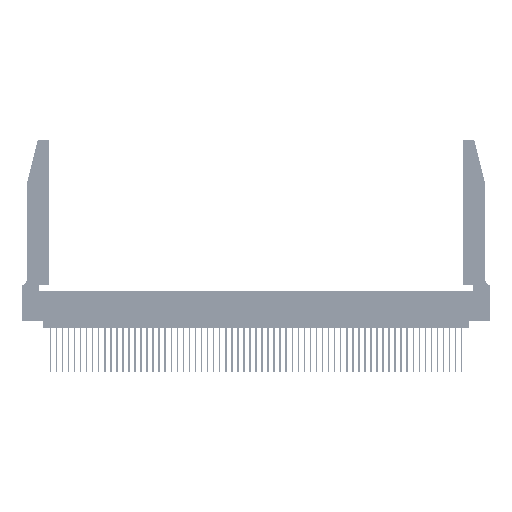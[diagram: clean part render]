
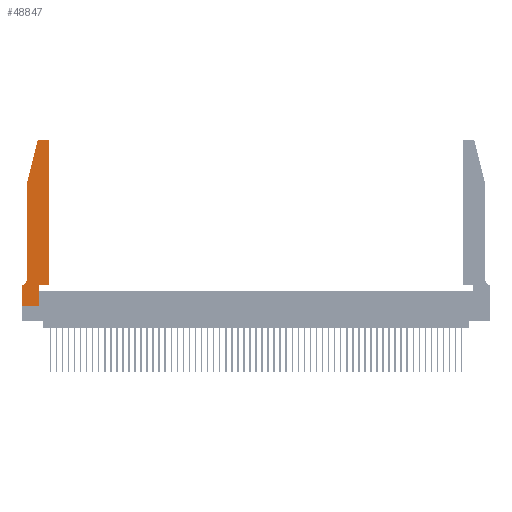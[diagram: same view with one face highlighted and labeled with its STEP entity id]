
A CAD part, top view. The second image highlights one B-rep face of the part: STEP entity #48847.
In plain terms, the highlighted planar face has unit normal (0, 0, 1).
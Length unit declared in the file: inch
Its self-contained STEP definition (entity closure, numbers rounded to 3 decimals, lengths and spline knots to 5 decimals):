
#72 = DIRECTION ( 'NONE',  ( 0., 0., 1. ) ) ;
#835 = CARTESIAN_POINT ( 'NONE',  ( 0.0755, 2., 0.37 ) ) ;
#942 = ORIENTED_EDGE ( 'NONE', *, *, #16438, .T. ) ;
#1132 = ORIENTED_EDGE ( 'NONE', *, *, #42555, .T. ) ;
#1268 = CIRCLE ( 'NONE', #54302, 0.03 ) ;
#1306 = DIRECTION ( 'NONE',  ( -1., 0., 0. ) ) ;
#1965 = CARTESIAN_POINT ( 'NONE',  ( 0.0755, 2., 0.37 ) ) ;
#4130 = ORIENTED_EDGE ( 'NONE', *, *, #50214, .T. ) ;
#4265 = CARTESIAN_POINT ( 'NONE',  ( 0.0055, 0.35, 0.37 ) ) ;
#4312 = VECTOR ( 'NONE', #8279, 39.37008 ) ;
#4739 = DIRECTION ( 'NONE',  ( 1., 0., 0. ) ) ;
#5356 = CARTESIAN_POINT ( 'NONE',  ( 0.4505, 0.35, 0.37 ) ) ;
#5868 = CARTESIAN_POINT ( 'NONE',  ( 0.2605, 2.75, 0.37 ) ) ;
#6295 = DIRECTION ( 'NONE',  ( 1., 0., 0. ) ) ;
#6496 = EDGE_CURVE ( 'NONE', #35958, #31170, #50195, .T. ) ;
#7111 = DIRECTION ( 'NONE',  ( 0., 1., 0. ) ) ;
#7503 = VECTOR ( 'NONE', #12842, 39.37008 ) ;
#8279 = DIRECTION ( 'NONE',  ( 0., -1., 0. ) ) ;
#8580 = DIRECTION ( 'NONE',  ( 1., 0., 0. ) ) ;
#9675 = EDGE_CURVE ( 'NONE', #44584, #35958, #25806, .T. ) ;
#10403 = ORIENTED_EDGE ( 'NONE', *, *, #6496, .T. ) ;
#10799 = VERTEX_POINT ( 'NONE', #4265 ) ;
#10897 = VERTEX_POINT ( 'NONE', #51812 ) ;
#11617 = VERTEX_POINT ( 'NONE', #24992 ) ;
#12486 = CARTESIAN_POINT ( 'NONE',  ( 0.4505, 0.35, 0.37 ) ) ;
#12708 = CARTESIAN_POINT ( 'NONE',  ( 0.4205, 2.72, 0.37 ) ) ;
#12842 = DIRECTION ( 'NONE',  ( 1., 0., 0. ) ) ;
#13895 = VERTEX_POINT ( 'NONE', #17860 ) ;
#15445 = DIRECTION ( 'NONE',  ( 0., 0., 1. ) ) ;
#15878 = DIRECTION ( 'NONE',  ( -1., 0., 0. ) ) ;
#16294 = ORIENTED_EDGE ( 'NONE', *, *, #53197, .T. ) ;
#16438 = EDGE_CURVE ( 'NONE', #42664, #13895, #1268, .T. ) ;
#17844 = VERTEX_POINT ( 'NONE', #43157 ) ;
#17860 = CARTESIAN_POINT ( 'NONE',  ( 0.4205, 2.75, 0.37 ) ) ;
#18050 = VECTOR ( 'NONE', #21969, 39.37008 ) ;
#18389 = EDGE_CURVE ( 'NONE', #47370, #10897, #19739, .T. ) ;
#18895 = LINE ( 'NONE', #12486, #7503 ) ;
#19739 = LINE ( 'NONE', #29807, #4312 ) ;
#20263 = EDGE_CURVE ( 'NONE', #31170, #10799, #22851, .T. ) ;
#21969 = DIRECTION ( 'NONE',  ( 0., -1., 0. ) ) ;
#22037 = AXIS2_PLACEMENT_3D ( 'NONE', #41635, #15445, #50071 ) ;
#22067 = CARTESIAN_POINT ( 'NONE',  ( 0.2865, 0., 0.37 ) ) ;
#22451 = VECTOR ( 'NONE', #35446, 39.37008 ) ;
#22851 = CIRCLE ( 'NONE', #25501, 0.07 ) ;
#22969 = FACE_OUTER_BOUND ( 'NONE', #47820, .T. ) ;
#23199 = ORIENTED_EDGE ( 'NONE', *, *, #49868, .T. ) ;
#23534 = VECTOR ( 'NONE', #6295, 39.37008 ) ;
#24973 = VECTOR ( 'NONE', #45069, 39.37008 ) ;
#24992 = CARTESIAN_POINT ( 'NONE',  ( 0.284, 2.75, 0.37 ) ) ;
#25501 = AXIS2_PLACEMENT_3D ( 'NONE', #52580, #31060, #1306 ) ;
#25806 = LINE ( 'NONE', #835, #22451 ) ;
#26675 = VECTOR ( 'NONE', #15878, 39.37008 ) ;
#26683 = VECTOR ( 'NONE', #7111, 39.37008 ) ;
#26853 = CARTESIAN_POINT ( 'NONE',  ( 0.0755, 2., 0.37 ) ) ;
#27468 = CARTESIAN_POINT ( 'NONE',  ( 0., 0., 0.37 ) ) ;
#28060 = CARTESIAN_POINT ( 'NONE',  ( 0.2865, 0.35, 0.37 ) ) ;
#28286 = LINE ( 'NONE', #27468, #23534 ) ;
#29106 = VERTEX_POINT ( 'NONE', #22067 ) ;
#29641 = LINE ( 'NONE', #28060, #24973 ) ;
#29807 = CARTESIAN_POINT ( 'NONE',  ( 0., 0., 0.37 ) ) ;
#30621 = CIRCLE ( 'NONE', #35798, 0.03 ) ;
#30904 = ORIENTED_EDGE ( 'NONE', *, *, #36757, .T. ) ;
#31060 = DIRECTION ( 'NONE',  ( 0., 0., -1. ) ) ;
#31170 = VERTEX_POINT ( 'NONE', #37018 ) ;
#32678 = LINE ( 'NONE', #49799, #26683 ) ;
#33031 = CARTESIAN_POINT ( 'NONE',  ( 0.25487, 2.72718, 0.37 ) ) ;
#35446 = DIRECTION ( 'NONE',  ( -0.239, -0.971, 0. ) ) ;
#35798 = AXIS2_PLACEMENT_3D ( 'NONE', #51362, #72, #4739 ) ;
#35958 = VERTEX_POINT ( 'NONE', #1965 ) ;
#36170 = VECTOR ( 'NONE', #49479, 39.37008 ) ;
#36615 = CARTESIAN_POINT ( 'NONE',  ( 0.4505, 2.72, 0.37 ) ) ;
#36757 = EDGE_CURVE ( 'NONE', #39988, #42664, #32678, .T. ) ;
#37018 = CARTESIAN_POINT ( 'NONE',  ( 0.0755, 0.42, 0.37 ) ) ;
#38790 = CARTESIAN_POINT ( 'NONE',  ( 0., 0.35, 0.37 ) ) ;
#39580 = ORIENTED_EDGE ( 'NONE', *, *, #20263, .T. ) ;
#39988 = VERTEX_POINT ( 'NONE', #5356 ) ;
#41144 = ORIENTED_EDGE ( 'NONE', *, *, #51449, .T. ) ;
#41635 = CARTESIAN_POINT ( 'NONE',  ( 0., 0.35, 0.37 ) ) ;
#42555 = EDGE_CURVE ( 'NONE', #10897, #29106, #28286, .T. ) ;
#42664 = VERTEX_POINT ( 'NONE', #36615 ) ;
#43157 = CARTESIAN_POINT ( 'NONE',  ( 0.2865, 0.35, 0.37 ) ) ;
#43425 = LINE ( 'NONE', #49182, #26675 ) ;
#44417 = EDGE_CURVE ( 'NONE', #10799, #47370, #43425, .T. ) ;
#44584 = VERTEX_POINT ( 'NONE', #33031 ) ;
#45069 = DIRECTION ( 'NONE',  ( 0., 1., 0. ) ) ;
#45567 = PLANE ( 'NONE',  #22037 ) ;
#46537 = ORIENTED_EDGE ( 'NONE', *, *, #18389, .T. ) ;
#47332 = DIRECTION ( 'NONE',  ( 0., 0., 1. ) ) ;
#47370 = VERTEX_POINT ( 'NONE', #38790 ) ;
#47820 = EDGE_LOOP ( 'NONE', ( #41144, #16294, #49164, #10403, #39580, #49088, #46537, #1132, #23199, #4130, #30904, #942 ) ) ;
#48847 = ADVANCED_FACE ( 'NONE', ( #22969 ), #45567, .T. ) ;
#49088 = ORIENTED_EDGE ( 'NONE', *, *, #44417, .T. ) ;
#49164 = ORIENTED_EDGE ( 'NONE', *, *, #9675, .T. ) ;
#49182 = CARTESIAN_POINT ( 'NONE',  ( 0.0755, 0.35, 0.37 ) ) ;
#49479 = DIRECTION ( 'NONE',  ( -1., 0., 0. ) ) ;
#49597 = LINE ( 'NONE', #5868, #36170 ) ;
#49799 = CARTESIAN_POINT ( 'NONE',  ( 0.4505, 0.35, 0.37 ) ) ;
#49868 = EDGE_CURVE ( 'NONE', #29106, #17844, #29641, .T. ) ;
#50071 = DIRECTION ( 'NONE',  ( 1., 0., 0. ) ) ;
#50195 = LINE ( 'NONE', #26853, #18050 ) ;
#50214 = EDGE_CURVE ( 'NONE', #17844, #39988, #18895, .T. ) ;
#51362 = CARTESIAN_POINT ( 'NONE',  ( 0.284, 2.72, 0.37 ) ) ;
#51449 = EDGE_CURVE ( 'NONE', #13895, #11617, #49597, .T. ) ;
#51812 = CARTESIAN_POINT ( 'NONE',  ( 0., 0., 0.37 ) ) ;
#52580 = CARTESIAN_POINT ( 'NONE',  ( 0.0055, 0.42, 0.37 ) ) ;
#53197 = EDGE_CURVE ( 'NONE', #11617, #44584, #30621, .T. ) ;
#54302 = AXIS2_PLACEMENT_3D ( 'NONE', #12708, #47332, #8580 ) ;
